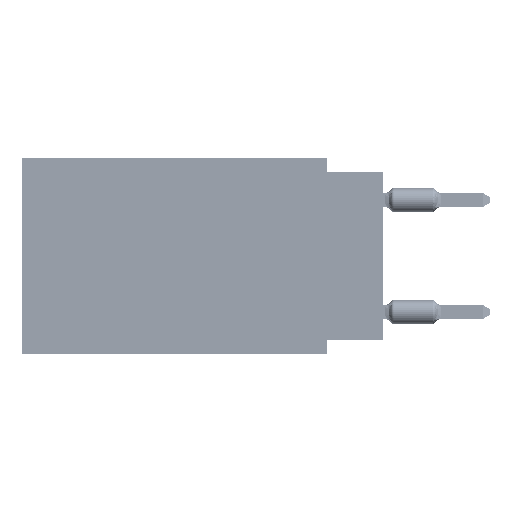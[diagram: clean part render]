
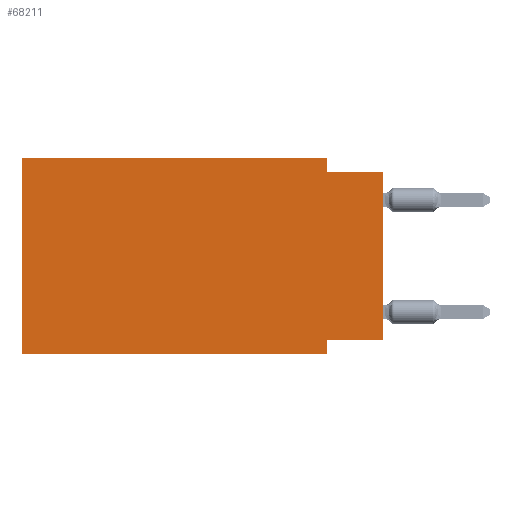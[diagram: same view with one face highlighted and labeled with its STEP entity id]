
A CAD part, left-side view. The second image highlights one B-rep face of the part: STEP entity #68211.
In plain terms, the highlighted planar face has unit normal (-1, 0, 0).
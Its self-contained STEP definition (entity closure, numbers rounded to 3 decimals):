
#1490 = VECTOR ( 'NONE', #52479, 1000. ) ;
#1641 = FACE_OUTER_BOUND ( 'NONE', #52285, .T. ) ;
#4053 = CARTESIAN_POINT ( 'NONE',  ( 0., 2.54, -8.255 ) ) ;
#4678 = VECTOR ( 'NONE', #46537, 1000. ) ;
#4871 = LINE ( 'NONE', #11076, #8949 ) ;
#4940 = CARTESIAN_POINT ( 'NONE',  ( 0., 16.383, -8.89 ) ) ;
#5741 = DIRECTION ( 'NONE',  ( 0., -1., 0. ) ) ;
#6445 = DIRECTION ( 'NONE',  ( 0., 0., -1. ) ) ;
#7440 = EDGE_CURVE ( 'NONE', #29043, #58206, #39760, .T. ) ;
#7556 = CARTESIAN_POINT ( 'NONE',  ( 0., 0., -0.635 ) ) ;
#7849 = LINE ( 'NONE', #13687, #1490 ) ;
#7885 = CARTESIAN_POINT ( 'NONE',  ( 0., 0., 0. ) ) ;
#8128 = VERTEX_POINT ( 'NONE', #4053 ) ;
#8949 = VECTOR ( 'NONE', #54270, 1000. ) ;
#11076 = CARTESIAN_POINT ( 'NONE',  ( 0., 2.54, -8.89 ) ) ;
#13687 = CARTESIAN_POINT ( 'NONE',  ( 0., 16.383, 0. ) ) ;
#13947 = CARTESIAN_POINT ( 'NONE',  ( 0., 16.383, 0. ) ) ;
#16890 = ORIENTED_EDGE ( 'NONE', *, *, #42025, .F. ) ;
#17733 = EDGE_CURVE ( 'NONE', #43094, #58206, #57992, .T. ) ;
#21135 = VECTOR ( 'NONE', #38079, 1000. ) ;
#22903 = CARTESIAN_POINT ( 'NONE',  ( 0., 2.54, 0. ) ) ;
#24300 = CARTESIAN_POINT ( 'NONE',  ( 0., 2.54, -8.89 ) ) ;
#24726 = VECTOR ( 'NONE', #6445, 1000. ) ;
#25465 = EDGE_CURVE ( 'NONE', #57303, #68114, #38328, .T. ) ;
#29043 = VERTEX_POINT ( 'NONE', #33790 ) ;
#31139 = ORIENTED_EDGE ( 'NONE', *, *, #37107, .F. ) ;
#32936 = CARTESIAN_POINT ( 'NONE',  ( 0., 0., -8.255 ) ) ;
#33528 = VECTOR ( 'NONE', #5741, 1000. ) ;
#33790 = CARTESIAN_POINT ( 'NONE',  ( 0., 2.54, -0.635 ) ) ;
#34622 = CARTESIAN_POINT ( 'NONE',  ( 0., 0., -0.635 ) ) ;
#35552 = LINE ( 'NONE', #13947, #4678 ) ;
#37107 = EDGE_CURVE ( 'NONE', #40172, #29043, #66777, .T. ) ;
#37944 = EDGE_CURVE ( 'NONE', #57303, #65938, #7849, .T. ) ;
#38079 = DIRECTION ( 'NONE',  ( 0., 1., 0. ) ) ;
#38328 = LINE ( 'NONE', #44182, #42189 ) ;
#39760 = LINE ( 'NONE', #34622, #33528 ) ;
#40172 = VERTEX_POINT ( 'NONE', #70177 ) ;
#42025 = EDGE_CURVE ( 'NONE', #43094, #8128, #61087, .T. ) ;
#42189 = VECTOR ( 'NONE', #42743, 1000. ) ;
#42743 = DIRECTION ( 'NONE',  ( 0., -1., 0. ) ) ;
#43094 = VERTEX_POINT ( 'NONE', #54192 ) ;
#44182 = CARTESIAN_POINT ( 'NONE',  ( 0., 16.383, -8.89 ) ) ;
#44649 = PLANE ( 'NONE',  #47274 ) ;
#46537 = DIRECTION ( 'NONE',  ( 0., -1., 0. ) ) ;
#46778 = ORIENTED_EDGE ( 'NONE', *, *, #17733, .T. ) ;
#46870 = EDGE_CURVE ( 'NONE', #8128, #68114, #4871, .T. ) ;
#47274 = AXIS2_PLACEMENT_3D ( 'NONE', #69978, #70708, #47716 ) ;
#47716 = DIRECTION ( 'NONE',  ( 0., 0., -1. ) ) ;
#49176 = VECTOR ( 'NONE', #56904, 1000. ) ;
#52285 = EDGE_LOOP ( 'NONE', ( #46778, #71788, #31139, #54847, #55127, #60364, #71180, #16890 ) ) ;
#52479 = DIRECTION ( 'NONE',  ( 0., 0., 1. ) ) ;
#54192 = CARTESIAN_POINT ( 'NONE',  ( 0., 0., -8.255 ) ) ;
#54270 = DIRECTION ( 'NONE',  ( 0., 0., -1. ) ) ;
#54847 = ORIENTED_EDGE ( 'NONE', *, *, #60276, .F. ) ;
#55127 = ORIENTED_EDGE ( 'NONE', *, *, #37944, .F. ) ;
#56904 = DIRECTION ( 'NONE',  ( 0., 0., 1. ) ) ;
#57303 = VERTEX_POINT ( 'NONE', #4940 ) ;
#57992 = LINE ( 'NONE', #7885, #49176 ) ;
#58206 = VERTEX_POINT ( 'NONE', #7556 ) ;
#60276 = EDGE_CURVE ( 'NONE', #65938, #40172, #35552, .T. ) ;
#60364 = ORIENTED_EDGE ( 'NONE', *, *, #25465, .T. ) ;
#61087 = LINE ( 'NONE', #32936, #21135 ) ;
#65938 = VERTEX_POINT ( 'NONE', #67974 ) ;
#66777 = LINE ( 'NONE', #22903, #24726 ) ;
#67974 = CARTESIAN_POINT ( 'NONE',  ( 0., 16.383, 0. ) ) ;
#68114 = VERTEX_POINT ( 'NONE', #24300 ) ;
#68211 = ADVANCED_FACE ( 'NONE', ( #1641 ), #44649, .F. ) ;
#69978 = CARTESIAN_POINT ( 'NONE',  ( 0., 16.383, 0. ) ) ;
#70177 = CARTESIAN_POINT ( 'NONE',  ( 0., 2.54, 0. ) ) ;
#70708 = DIRECTION ( 'NONE',  ( 1., 0., 0. ) ) ;
#71180 = ORIENTED_EDGE ( 'NONE', *, *, #46870, .F. ) ;
#71788 = ORIENTED_EDGE ( 'NONE', *, *, #7440, .F. ) ;
